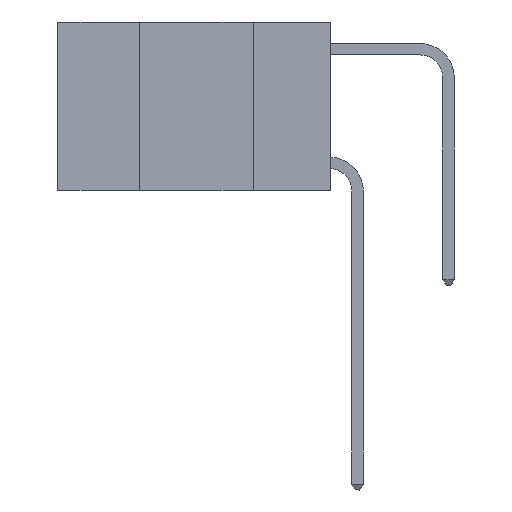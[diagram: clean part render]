
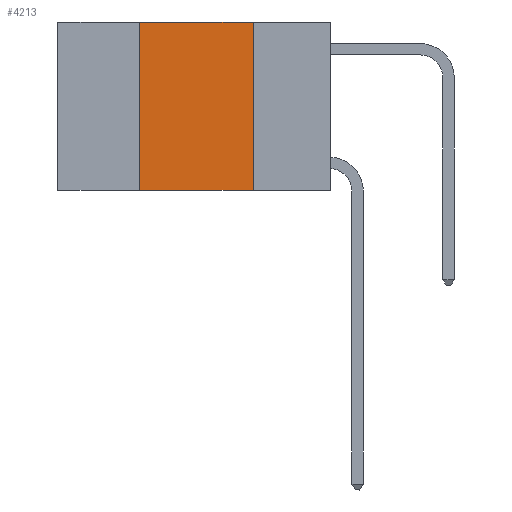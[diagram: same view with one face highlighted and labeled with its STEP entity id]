
A CAD part, left-side view. The second image highlights one B-rep face of the part: STEP entity #4213.
In plain terms, the highlighted planar face has unit normal (-1, 0, 0).
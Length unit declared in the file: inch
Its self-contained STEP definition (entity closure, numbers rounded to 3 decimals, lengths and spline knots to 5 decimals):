
#357 = CARTESIAN_POINT ( 'NONE',  ( 0., 0.6, 0. ) ) ;
#583 = EDGE_LOOP ( 'NONE', ( #1314, #4121, #6792, #9293 ) ) ;
#743 = PLANE ( 'NONE',  #4163 ) ;
#1314 = ORIENTED_EDGE ( 'NONE', *, *, #10686, .F. ) ;
#2625 = LINE ( 'NONE', #4307, #12470 ) ;
#2931 = LINE ( 'NONE', #9184, #7589 ) ;
#2989 = DIRECTION ( 'NONE',  ( 0., 0., -1. ) ) ;
#3104 = CARTESIAN_POINT ( 'NONE',  ( 0., 0.6, -0.37 ) ) ;
#3216 = VERTEX_POINT ( 'NONE', #8235 ) ;
#3252 = LINE ( 'NONE', #3104, #10925 ) ;
#3356 = DIRECTION ( 'NONE',  ( 0., 0., -1. ) ) ;
#3634 = DIRECTION ( 'NONE',  ( 0., -1., 0. ) ) ;
#3926 = CARTESIAN_POINT ( 'NONE',  ( 0., 0.17, 0. ) ) ;
#4121 = ORIENTED_EDGE ( 'NONE', *, *, #12700, .F. ) ;
#4163 = AXIS2_PLACEMENT_3D ( 'NONE', #4948, #8845, #2989 ) ;
#4213 = ADVANCED_FACE ( 'NONE', ( #9416 ), #743, .F. ) ;
#4307 = CARTESIAN_POINT ( 'NONE',  ( 0., 0.42, 0. ) ) ;
#4948 = CARTESIAN_POINT ( 'NONE',  ( 0., 0.6, 0. ) ) ;
#5948 = VERTEX_POINT ( 'NONE', #6363 ) ;
#6342 = DIRECTION ( 'NONE',  ( 0., 0., 1. ) ) ;
#6363 = CARTESIAN_POINT ( 'NONE',  ( 0., 0.17, -0.37 ) ) ;
#6751 = CARTESIAN_POINT ( 'NONE',  ( 0., 0.42, 0. ) ) ;
#6792 = ORIENTED_EDGE ( 'NONE', *, *, #10666, .F. ) ;
#7589 = VECTOR ( 'NONE', #3356, 39.37008 ) ;
#8054 = VERTEX_POINT ( 'NONE', #6751 ) ;
#8235 = CARTESIAN_POINT ( 'NONE',  ( 0., 0.42, -0.37 ) ) ;
#8297 = VERTEX_POINT ( 'NONE', #3926 ) ;
#8845 = DIRECTION ( 'NONE',  ( 1., 0., 0. ) ) ;
#9184 = CARTESIAN_POINT ( 'NONE',  ( 0., 0.17, 0. ) ) ;
#9293 = ORIENTED_EDGE ( 'NONE', *, *, #10523, .T. ) ;
#9416 = FACE_OUTER_BOUND ( 'NONE', #583, .T. ) ;
#9741 = VECTOR ( 'NONE', #3634, 39.37008 ) ;
#9932 = DIRECTION ( 'NONE',  ( 0., -1., 0. ) ) ;
#10523 = EDGE_CURVE ( 'NONE', #3216, #5948, #3252, .T. ) ;
#10666 = EDGE_CURVE ( 'NONE', #3216, #8054, #2625, .T. ) ;
#10686 = EDGE_CURVE ( 'NONE', #8297, #5948, #2931, .T. ) ;
#10925 = VECTOR ( 'NONE', #9932, 39.37008 ) ;
#12170 = LINE ( 'NONE', #357, #9741 ) ;
#12470 = VECTOR ( 'NONE', #6342, 39.37008 ) ;
#12700 = EDGE_CURVE ( 'NONE', #8054, #8297, #12170, .T. ) ;
